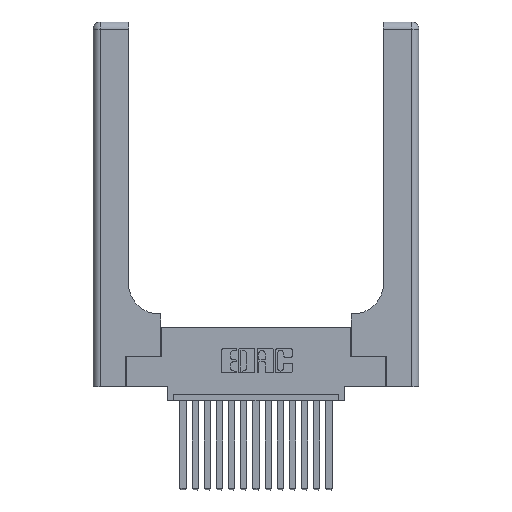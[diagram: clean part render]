
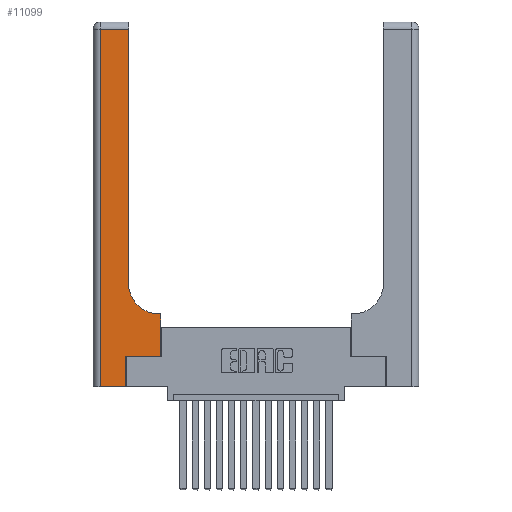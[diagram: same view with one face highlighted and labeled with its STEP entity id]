
A CAD part, top view. The second image highlights one B-rep face of the part: STEP entity #11099.
In plain terms, the highlighted planar face has unit normal (0, 0, 1).
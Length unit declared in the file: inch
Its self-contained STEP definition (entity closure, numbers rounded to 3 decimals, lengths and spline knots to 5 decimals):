
#196 = DIRECTION ( 'NONE',  ( 0., 1., 0. ) ) ;
#219 = CARTESIAN_POINT ( 'NONE',  ( 0.269, 0.25, 0.37 ) ) ;
#220 = CARTESIAN_POINT ( 'NONE',  ( 0.269, 0., 0.37 ) ) ;
#392 = DIRECTION ( 'NONE',  ( 0., 0., -1. ) ) ;
#472 = EDGE_CURVE ( 'NONE', #5448, #4735, #1452, .T. ) ;
#1029 = CARTESIAN_POINT ( 'NONE',  ( 0.5585, 0.6, 0.37 ) ) ;
#1424 = FACE_OUTER_BOUND ( 'NONE', #10483, .T. ) ;
#1452 = LINE ( 'NONE', #11315, #1904 ) ;
#1620 = AXIS2_PLACEMENT_3D ( 'NONE', #6171, #392, #16393 ) ;
#1740 = LINE ( 'NONE', #11620, #8352 ) ;
#1904 = VECTOR ( 'NONE', #7000, 39.37008 ) ;
#1969 = VERTEX_POINT ( 'NONE', #8465 ) ;
#2132 = VERTEX_POINT ( 'NONE', #3977 ) ;
#2450 = DIRECTION ( 'NONE',  ( 0., 1., 0. ) ) ;
#2742 = VERTEX_POINT ( 'NONE', #3690 ) ;
#2815 = VERTEX_POINT ( 'NONE', #1029 ) ;
#2857 = DIRECTION ( 'NONE',  ( 1., 0., 0. ) ) ;
#2893 = CARTESIAN_POINT ( 'NONE',  ( 0.5585, 0.25, 0.37 ) ) ;
#3126 = EDGE_CURVE ( 'NONE', #2132, #2742, #12502, .T. ) ;
#3225 = VECTOR ( 'NONE', #8528, 39.37008 ) ;
#3501 = LINE ( 'NONE', #12506, #18027 ) ;
#3571 = EDGE_CURVE ( 'NONE', #9312, #5448, #9698, .T. ) ;
#3690 = CARTESIAN_POINT ( 'NONE',  ( 0.2915, 0.85, 0.37 ) ) ;
#3865 = ORIENTED_EDGE ( 'NONE', *, *, #10976, .T. ) ;
#3977 = CARTESIAN_POINT ( 'NONE',  ( 0.5415, 0.6, 0.37 ) ) ;
#4047 = CARTESIAN_POINT ( 'NONE',  ( 0.269, 0.25, 0.37 ) ) ;
#4139 = DIRECTION ( 'NONE',  ( 0., -1., 0. ) ) ;
#4603 = CARTESIAN_POINT ( 'NONE',  ( 0.5585, 0.25, 0.37 ) ) ;
#4735 = VERTEX_POINT ( 'NONE', #219 ) ;
#5448 = VERTEX_POINT ( 'NONE', #220 ) ;
#5471 = DIRECTION ( 'NONE',  ( -1., 0., 0. ) ) ;
#5571 = CARTESIAN_POINT ( 'NONE',  ( 0.2915, 2.94, 0.37 ) ) ;
#5658 = DIRECTION ( 'NONE',  ( 0., 0., -1. ) ) ;
#5788 = VECTOR ( 'NONE', #8251, 39.37008 ) ;
#5903 = ORIENTED_EDGE ( 'NONE', *, *, #3571, .T. ) ;
#6171 = CARTESIAN_POINT ( 'NONE',  ( 0., 3., 0.37 ) ) ;
#6679 = EDGE_CURVE ( 'NONE', #2742, #8555, #3501, .T. ) ;
#7000 = DIRECTION ( 'NONE',  ( 0., 1., 0. ) ) ;
#7201 = EDGE_CURVE ( 'NONE', #4735, #14944, #9151, .T. ) ;
#7336 = LINE ( 'NONE', #4603, #13473 ) ;
#7460 = VECTOR ( 'NONE', #5471, 39.37008 ) ;
#7987 = EDGE_CURVE ( 'NONE', #2815, #2132, #9599, .T. ) ;
#8196 = ORIENTED_EDGE ( 'NONE', *, *, #3126, .T. ) ;
#8251 = DIRECTION ( 'NONE',  ( 1., 0., 0. ) ) ;
#8352 = VECTOR ( 'NONE', #4139, 39.37008 ) ;
#8465 = CARTESIAN_POINT ( 'NONE',  ( 0.06, 2.94, 0.37 ) ) ;
#8528 = DIRECTION ( 'NONE',  ( -1., 0., 0. ) ) ;
#8555 = VERTEX_POINT ( 'NONE', #5571 ) ;
#8643 = CARTESIAN_POINT ( 'NONE',  ( 0., 2.94, 0.37 ) ) ;
#8932 = VECTOR ( 'NONE', #13999, 39.37008 ) ;
#9151 = LINE ( 'NONE', #4047, #8932 ) ;
#9312 = VERTEX_POINT ( 'NONE', #11974 ) ;
#9599 = LINE ( 'NONE', #17204, #3225 ) ;
#9698 = LINE ( 'NONE', #16946, #5788 ) ;
#10438 = AXIS2_PLACEMENT_3D ( 'NONE', #17842, #5658, #2857 ) ;
#10483 = EDGE_LOOP ( 'NONE', ( #18590, #16732, #16138, #5903, #15208, #17302, #3865, #14052, #8196 ) ) ;
#10976 = EDGE_CURVE ( 'NONE', #14944, #2815, #7336, .T. ) ;
#11099 = ADVANCED_FACE ( 'NONE', ( #1424 ), #17836, .F. ) ;
#11118 = LINE ( 'NONE', #8643, #7460 ) ;
#11315 = CARTESIAN_POINT ( 'NONE',  ( 0.269, 0., 0.37 ) ) ;
#11620 = CARTESIAN_POINT ( 'NONE',  ( 0.06, 3., 0.37 ) ) ;
#11974 = CARTESIAN_POINT ( 'NONE',  ( 0.06, 0., 0.37 ) ) ;
#12502 = CIRCLE ( 'NONE', #10438, 0.25 ) ;
#12506 = CARTESIAN_POINT ( 'NONE',  ( 0.2915, 3., 0.37 ) ) ;
#13473 = VECTOR ( 'NONE', #196, 39.37008 ) ;
#13999 = DIRECTION ( 'NONE',  ( 1., 0., 0. ) ) ;
#14052 = ORIENTED_EDGE ( 'NONE', *, *, #7987, .T. ) ;
#14376 = EDGE_CURVE ( 'NONE', #1969, #9312, #1740, .T. ) ;
#14944 = VERTEX_POINT ( 'NONE', #2893 ) ;
#15208 = ORIENTED_EDGE ( 'NONE', *, *, #472, .T. ) ;
#16138 = ORIENTED_EDGE ( 'NONE', *, *, #14376, .T. ) ;
#16393 = DIRECTION ( 'NONE',  ( -1., 0., 0. ) ) ;
#16732 = ORIENTED_EDGE ( 'NONE', *, *, #18290, .T. ) ;
#16946 = CARTESIAN_POINT ( 'NONE',  ( 0., 0., 0.37 ) ) ;
#17204 = CARTESIAN_POINT ( 'NONE',  ( 0.2915, 0.6, 0.37 ) ) ;
#17302 = ORIENTED_EDGE ( 'NONE', *, *, #7201, .T. ) ;
#17836 = PLANE ( 'NONE',  #1620 ) ;
#17842 = CARTESIAN_POINT ( 'NONE',  ( 0.5415, 0.85, 0.37 ) ) ;
#18027 = VECTOR ( 'NONE', #2450, 39.37008 ) ;
#18290 = EDGE_CURVE ( 'NONE', #8555, #1969, #11118, .T. ) ;
#18590 = ORIENTED_EDGE ( 'NONE', *, *, #6679, .T. ) ;
